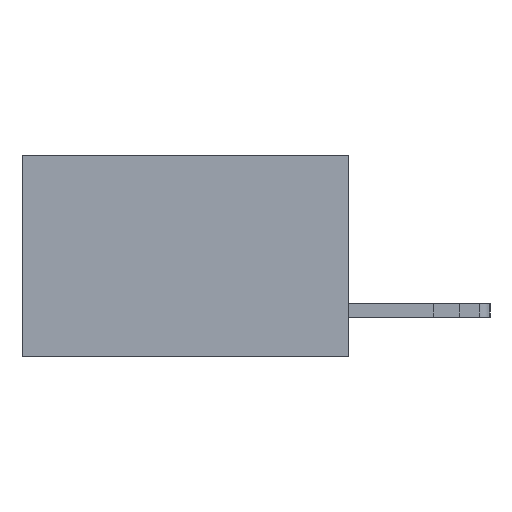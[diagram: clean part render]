
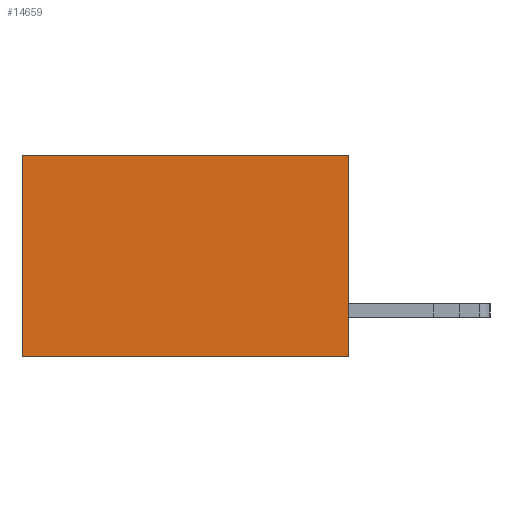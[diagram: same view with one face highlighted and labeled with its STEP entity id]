
A CAD part, left-side view. The second image highlights one B-rep face of the part: STEP entity #14659.
In plain terms, the highlighted planar face has unit normal (-1, 0, 0).
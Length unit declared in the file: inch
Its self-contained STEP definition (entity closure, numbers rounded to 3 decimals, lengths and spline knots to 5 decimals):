
#420 = CARTESIAN_POINT ( 'NONE',  ( 0.298, 0., 0. ) ) ;
#453 = DIRECTION ( 'NONE',  ( 0., 1., 0. ) ) ;
#646 = EDGE_CURVE ( 'NONE', #1898, #4618, #16434, .T. ) ;
#708 = EDGE_LOOP ( 'NONE', ( #11792, #11921, #8184, #6411 ) ) ;
#770 = CARTESIAN_POINT ( 'NONE',  ( 0.298, 0., 0. ) ) ;
#1168 = VECTOR ( 'NONE', #7320, 39.37008 ) ;
#1775 = VECTOR ( 'NONE', #9555, 39.37008 ) ;
#1898 = VERTEX_POINT ( 'NONE', #12410 ) ;
#1983 = FACE_OUTER_BOUND ( 'NONE', #708, .T. ) ;
#2152 = DIRECTION ( 'NONE',  ( 0., 0., -1. ) ) ;
#2196 = LINE ( 'NONE', #420, #1775 ) ;
#2725 = LINE ( 'NONE', #4323, #12273 ) ;
#4323 = CARTESIAN_POINT ( 'NONE',  ( 0.298, 0., -0.37 ) ) ;
#4618 = VERTEX_POINT ( 'NONE', #7302 ) ;
#6224 = VECTOR ( 'NONE', #453, 39.37008 ) ;
#6411 = ORIENTED_EDGE ( 'NONE', *, *, #646, .T. ) ;
#7302 = CARTESIAN_POINT ( 'NONE',  ( 0.298, 0.6, 0. ) ) ;
#7320 = DIRECTION ( 'NONE',  ( 0., 0., -1. ) ) ;
#7488 = CARTESIAN_POINT ( 'NONE',  ( 0.298, 0.6, 0. ) ) ;
#7606 = EDGE_CURVE ( 'NONE', #4618, #10467, #15377, .T. ) ;
#8184 = ORIENTED_EDGE ( 'NONE', *, *, #14484, .F. ) ;
#8670 = PLANE ( 'NONE',  #13302 ) ;
#9555 = DIRECTION ( 'NONE',  ( 0., 0., -1. ) ) ;
#9961 = DIRECTION ( 'NONE',  ( 1., 0., 0. ) ) ;
#10277 = VERTEX_POINT ( 'NONE', #10691 ) ;
#10303 = EDGE_CURVE ( 'NONE', #10277, #10467, #2725, .T. ) ;
#10467 = VERTEX_POINT ( 'NONE', #11126 ) ;
#10691 = CARTESIAN_POINT ( 'NONE',  ( 0.298, 0., -0.37 ) ) ;
#11126 = CARTESIAN_POINT ( 'NONE',  ( 0.298, 0.6, -0.37 ) ) ;
#11213 = CARTESIAN_POINT ( 'NONE',  ( 0.298, 0., 0. ) ) ;
#11792 = ORIENTED_EDGE ( 'NONE', *, *, #7606, .T. ) ;
#11921 = ORIENTED_EDGE ( 'NONE', *, *, #10303, .F. ) ;
#12076 = DIRECTION ( 'NONE',  ( 0., 1., 0. ) ) ;
#12273 = VECTOR ( 'NONE', #12076, 39.37008 ) ;
#12410 = CARTESIAN_POINT ( 'NONE',  ( 0.298, 0., 0. ) ) ;
#13302 = AXIS2_PLACEMENT_3D ( 'NONE', #11213, #9961, #2152 ) ;
#14484 = EDGE_CURVE ( 'NONE', #1898, #10277, #2196, .T. ) ;
#14659 = ADVANCED_FACE ( 'NONE', ( #1983 ), #8670, .F. ) ;
#15377 = LINE ( 'NONE', #7488, #1168 ) ;
#16434 = LINE ( 'NONE', #770, #6224 ) ;
